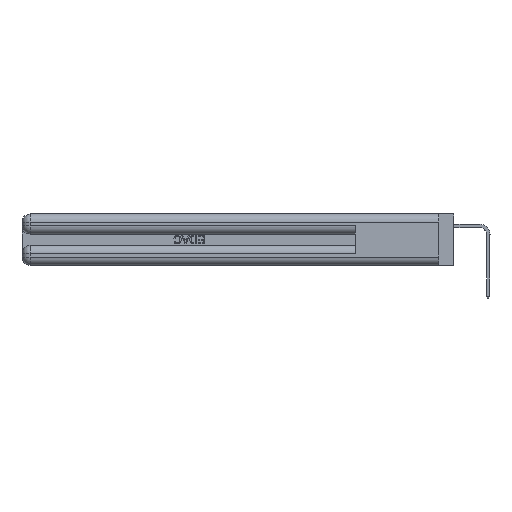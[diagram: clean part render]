
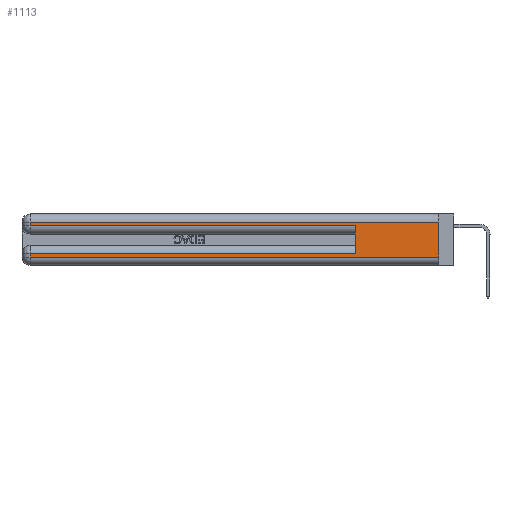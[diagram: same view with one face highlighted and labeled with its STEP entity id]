
A CAD part, left-side view. The second image highlights one B-rep face of the part: STEP entity #1113.
In plain terms, the highlighted planar face has unit normal (-1, 0, 0).
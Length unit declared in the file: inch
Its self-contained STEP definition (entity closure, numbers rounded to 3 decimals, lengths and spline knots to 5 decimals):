
#660 = VERTEX_POINT ( 'NONE', #7816 ) ;
#1113 = ADVANCED_FACE ( 'NONE', ( #1736 ), #6561, .F. ) ;
#1546 = VECTOR ( 'NONE', #31079, 39.37008 ) ;
#1736 = FACE_OUTER_BOUND ( 'NONE', #42768, .T. ) ;
#1891 = ORIENTED_EDGE ( 'NONE', *, *, #19670, .T. ) ;
#2234 = VERTEX_POINT ( 'NONE', #34347 ) ;
#2636 = LINE ( 'NONE', #10129, #1546 ) ;
#3216 = VERTEX_POINT ( 'NONE', #43716 ) ;
#3342 = LINE ( 'NONE', #20123, #11481 ) ;
#3610 = CARTESIAN_POINT ( 'NONE',  ( 0., 0., 0.31 ) ) ;
#6287 = ORIENTED_EDGE ( 'NONE', *, *, #28338, .T. ) ;
#6561 = PLANE ( 'NONE',  #29771 ) ;
#7816 = CARTESIAN_POINT ( 'NONE',  ( 0., 2.94, 0.085 ) ) ;
#7923 = VECTOR ( 'NONE', #10167, 39.37008 ) ;
#7958 = DIRECTION ( 'NONE',  ( 0., 1., 0. ) ) ;
#8318 = VERTEX_POINT ( 'NONE', #19561 ) ;
#9449 = LINE ( 'NONE', #20413, #24627 ) ;
#9535 = VECTOR ( 'NONE', #18496, 39.37008 ) ;
#9590 = CARTESIAN_POINT ( 'NONE',  ( 0., 2.94, 0.285 ) ) ;
#10036 = DIRECTION ( 'NONE',  ( 1., 0., 0. ) ) ;
#10129 = CARTESIAN_POINT ( 'NONE',  ( 0., 2.94, 0.37 ) ) ;
#10167 = DIRECTION ( 'NONE',  ( 0., 0., 1. ) ) ;
#10769 = CARTESIAN_POINT ( 'NONE',  ( 0., 0.6, 0.285 ) ) ;
#11481 = VECTOR ( 'NONE', #40941, 39.37008 ) ;
#12271 = VERTEX_POINT ( 'NONE', #3610 ) ;
#13038 = CARTESIAN_POINT ( 'NONE',  ( 0., 0., 0.31 ) ) ;
#13680 = EDGE_CURVE ( 'NONE', #37867, #18232, #35598, .T. ) ;
#13777 = ORIENTED_EDGE ( 'NONE', *, *, #34264, .F. ) ;
#14733 = CARTESIAN_POINT ( 'NONE',  ( 0., 0.6, 0.085 ) ) ;
#15269 = VECTOR ( 'NONE', #28319, 39.37008 ) ;
#17604 = ORIENTED_EDGE ( 'NONE', *, *, #28088, .T. ) ;
#17860 = CARTESIAN_POINT ( 'NONE',  ( 0., 0., 0.06 ) ) ;
#18232 = VERTEX_POINT ( 'NONE', #10769 ) ;
#18262 = CARTESIAN_POINT ( 'NONE',  ( 0., 0., 0.085 ) ) ;
#18496 = DIRECTION ( 'NONE',  ( 0., 0., -1. ) ) ;
#18644 = ORIENTED_EDGE ( 'NONE', *, *, #37233, .T. ) ;
#19561 = CARTESIAN_POINT ( 'NONE',  ( 0., 2.94, 0.06 ) ) ;
#19670 = EDGE_CURVE ( 'NONE', #2234, #39583, #2636, .T. ) ;
#20123 = CARTESIAN_POINT ( 'NONE',  ( 0., 0., 0.37 ) ) ;
#20413 = CARTESIAN_POINT ( 'NONE',  ( 0., 0., 0.285 ) ) ;
#21753 = EDGE_CURVE ( 'NONE', #660, #8318, #30179, .T. ) ;
#22469 = ORIENTED_EDGE ( 'NONE', *, *, #40894, .T. ) ;
#24627 = VECTOR ( 'NONE', #30853, 39.37008 ) ;
#27337 = CARTESIAN_POINT ( 'NONE',  ( 0., 0., 0.37 ) ) ;
#27476 = ORIENTED_EDGE ( 'NONE', *, *, #21753, .T. ) ;
#27478 = CARTESIAN_POINT ( 'NONE',  ( 0., 0.6, 0.145 ) ) ;
#28088 = EDGE_CURVE ( 'NONE', #12271, #2234, #44632, .T. ) ;
#28319 = DIRECTION ( 'NONE',  ( 0., -1., 0. ) ) ;
#28338 = EDGE_CURVE ( 'NONE', #8318, #3216, #42987, .T. ) ;
#29771 = AXIS2_PLACEMENT_3D ( 'NONE', #27337, #10036, #34318 ) ;
#30179 = LINE ( 'NONE', #42793, #9535 ) ;
#30853 = DIRECTION ( 'NONE',  ( 0., -1., 0. ) ) ;
#31079 = DIRECTION ( 'NONE',  ( 0., 0., -1. ) ) ;
#33427 = VECTOR ( 'NONE', #7958, 39.37008 ) ;
#34264 = EDGE_CURVE ( 'NONE', #12271, #3216, #3342, .T. ) ;
#34318 = DIRECTION ( 'NONE',  ( 0., 0., -1. ) ) ;
#34347 = CARTESIAN_POINT ( 'NONE',  ( 0., 2.94, 0.31 ) ) ;
#35598 = LINE ( 'NONE', #27478, #7923 ) ;
#37233 = EDGE_CURVE ( 'NONE', #37867, #660, #42691, .T. ) ;
#37867 = VERTEX_POINT ( 'NONE', #14733 ) ;
#39583 = VERTEX_POINT ( 'NONE', #9590 ) ;
#40894 = EDGE_CURVE ( 'NONE', #39583, #18232, #9449, .T. ) ;
#40941 = DIRECTION ( 'NONE',  ( 0., 0., -1. ) ) ;
#40984 = DIRECTION ( 'NONE',  ( 0., 1., 0. ) ) ;
#42691 = LINE ( 'NONE', #18262, #33427 ) ;
#42768 = EDGE_LOOP ( 'NONE', ( #13777, #17604, #1891, #22469, #43725, #18644, #27476, #6287 ) ) ;
#42793 = CARTESIAN_POINT ( 'NONE',  ( 0., 2.94, 0.37 ) ) ;
#42987 = LINE ( 'NONE', #17860, #15269 ) ;
#43551 = VECTOR ( 'NONE', #40984, 39.37008 ) ;
#43716 = CARTESIAN_POINT ( 'NONE',  ( 0., 0., 0.06 ) ) ;
#43725 = ORIENTED_EDGE ( 'NONE', *, *, #13680, .F. ) ;
#44632 = LINE ( 'NONE', #13038, #43551 ) ;
